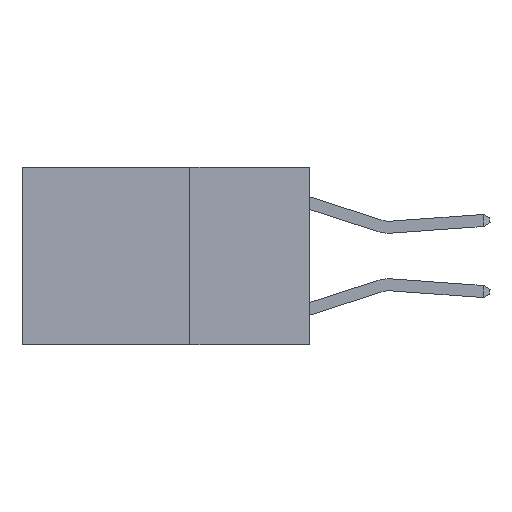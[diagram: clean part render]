
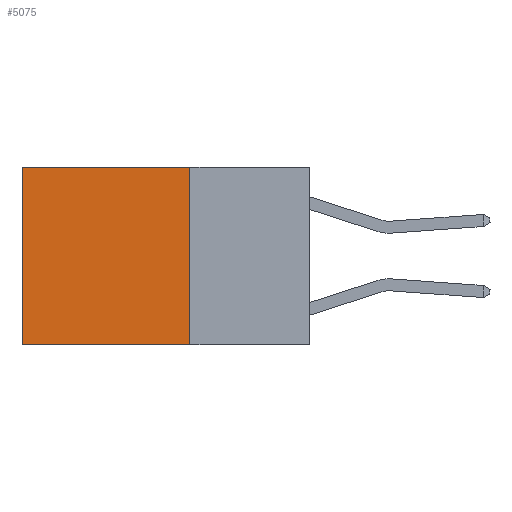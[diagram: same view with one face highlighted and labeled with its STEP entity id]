
A CAD part, left-side view. The second image highlights one B-rep face of the part: STEP entity #5075.
In plain terms, the highlighted planar face has unit normal (-1, 0, 0).
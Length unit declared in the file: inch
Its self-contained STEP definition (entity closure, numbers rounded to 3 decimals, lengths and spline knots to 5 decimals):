
#39 = DIRECTION ( 'NONE',  ( 1., 0., 0. ) ) ;
#263 = LINE ( 'NONE', #9079, #5174 ) ;
#932 = VECTOR ( 'NONE', #5154, 39.37008 ) ;
#2842 = FACE_OUTER_BOUND ( 'NONE', #14639, .T. ) ;
#3437 = VERTEX_POINT ( 'NONE', #6623 ) ;
#3572 = ORIENTED_EDGE ( 'NONE', *, *, #13152, .T. ) ;
#4639 = CARTESIAN_POINT ( 'NONE',  ( 0.2625, 0.25, -0.37 ) ) ;
#5053 = VERTEX_POINT ( 'NONE', #13314 ) ;
#5075 = ADVANCED_FACE ( 'NONE', ( #2842 ), #8949, .F. ) ;
#5154 = DIRECTION ( 'NONE',  ( 0., 0., -1. ) ) ;
#5174 = VECTOR ( 'NONE', #7621, 39.37008 ) ;
#5373 = AXIS2_PLACEMENT_3D ( 'NONE', #13217, #39, #19123 ) ;
#5482 = EDGE_CURVE ( 'NONE', #8616, #5053, #14746, .T. ) ;
#5905 = LINE ( 'NONE', #4639, #9277 ) ;
#6104 = DIRECTION ( 'NONE',  ( 0., 1., 0. ) ) ;
#6476 = CARTESIAN_POINT ( 'NONE',  ( 0.2625, 0.6, 0. ) ) ;
#6497 = CARTESIAN_POINT ( 'NONE',  ( 0.2625, 0.25, 0. ) ) ;
#6623 = CARTESIAN_POINT ( 'NONE',  ( 0.2625, 0.6, -0.37 ) ) ;
#7621 = DIRECTION ( 'NONE',  ( 0., 1., 0. ) ) ;
#8410 = ORIENTED_EDGE ( 'NONE', *, *, #14987, .T. ) ;
#8616 = VERTEX_POINT ( 'NONE', #6497 ) ;
#8949 = PLANE ( 'NONE',  #5373 ) ;
#9022 = VERTEX_POINT ( 'NONE', #6476 ) ;
#9079 = CARTESIAN_POINT ( 'NONE',  ( 0.2625, 0.25, 0. ) ) ;
#9277 = VECTOR ( 'NONE', #6104, 39.37008 ) ;
#9444 = CARTESIAN_POINT ( 'NONE',  ( 0.2625, 0.6, 0. ) ) ;
#10470 = CARTESIAN_POINT ( 'NONE',  ( 0.2625, 0.25, 0. ) ) ;
#11592 = VECTOR ( 'NONE', #13385, 39.37008 ) ;
#12264 = ORIENTED_EDGE ( 'NONE', *, *, #5482, .F. ) ;
#13152 = EDGE_CURVE ( 'NONE', #8616, #9022, #263, .T. ) ;
#13217 = CARTESIAN_POINT ( 'NONE',  ( 0.2625, 0.25, 0. ) ) ;
#13314 = CARTESIAN_POINT ( 'NONE',  ( 0.2625, 0.25, -0.37 ) ) ;
#13385 = DIRECTION ( 'NONE',  ( 0., 0., -1. ) ) ;
#14639 = EDGE_LOOP ( 'NONE', ( #8410, #18637, #12264, #3572 ) ) ;
#14746 = LINE ( 'NONE', #10470, #11592 ) ;
#14987 = EDGE_CURVE ( 'NONE', #9022, #3437, #15538, .T. ) ;
#15538 = LINE ( 'NONE', #9444, #932 ) ;
#18419 = EDGE_CURVE ( 'NONE', #5053, #3437, #5905, .T. ) ;
#18637 = ORIENTED_EDGE ( 'NONE', *, *, #18419, .F. ) ;
#19123 = DIRECTION ( 'NONE',  ( 0., 0., -1. ) ) ;
